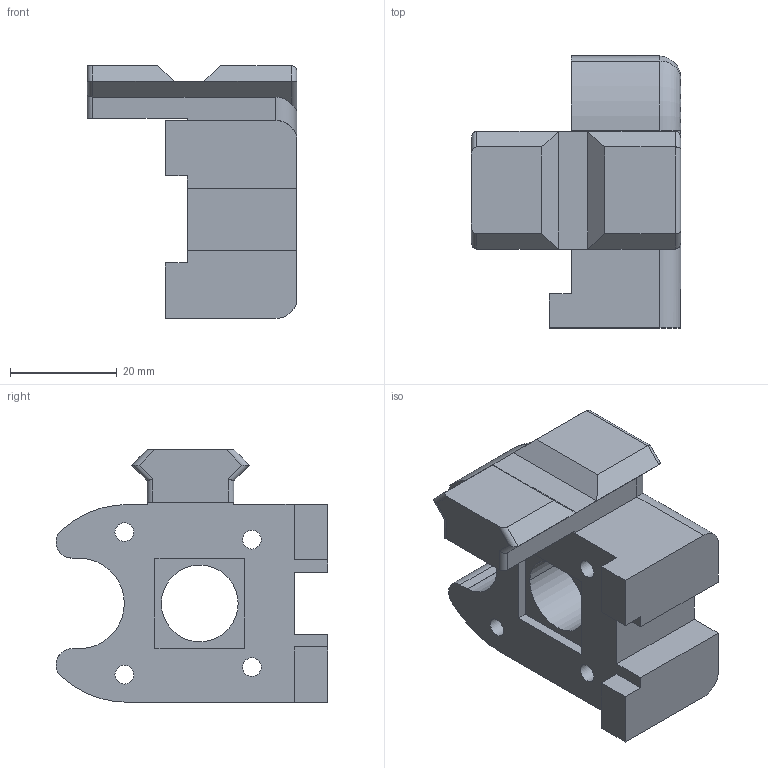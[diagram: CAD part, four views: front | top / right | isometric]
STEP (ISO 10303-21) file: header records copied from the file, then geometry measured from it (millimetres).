
FILE_DESCRIPTION (( 'STEP AP203' ), '1' );
FILE_NAME ('WTF-9_hillbilly_barrel_retainer_rail.STEP', '2020-05-09T08:52:04', ( '' ), ( '' ), 'SwSTEP 2.0', 'SolidWorks 2016', '' );
FILE_SCHEMA (( 'CONFIG_CONTROL_DESIGN' ));
Length unit declared in the file: millimetre
Products named in the file (2): WTF-9_hillbilly_barrel_retainer_rail; WTF HILLBILLY FINAL_14
Assembly tree (1 placements, depth 2):
  WTF-9_hillbilly_barrel_retainer_rail
    WTF HILLBILLY FINAL_14
Bounding box: 39.28 x 50.94 x 47.36 mm (x, y, z)
Volume: 34739.6 mm3; surface area: 10645.1 mm2
Topology: 1 solids, 1 shells, 78 faces, 210 edges, 135 vertices
Faces by surface type: plane 42, cylinder 30, torus 4, bspline 2
Full cylindrical faces by diameter (mm): 3.5 x4
Entity records: 2898 total; most frequent: CARTESIAN_POINT 795, ORIENTED_EDGE 412, DIRECTION 371, EDGE_CURVE 206, LINE 139, VECTOR 139, VERTEX_POINT 135, AXIS2_PLACEMENT_3D 116
